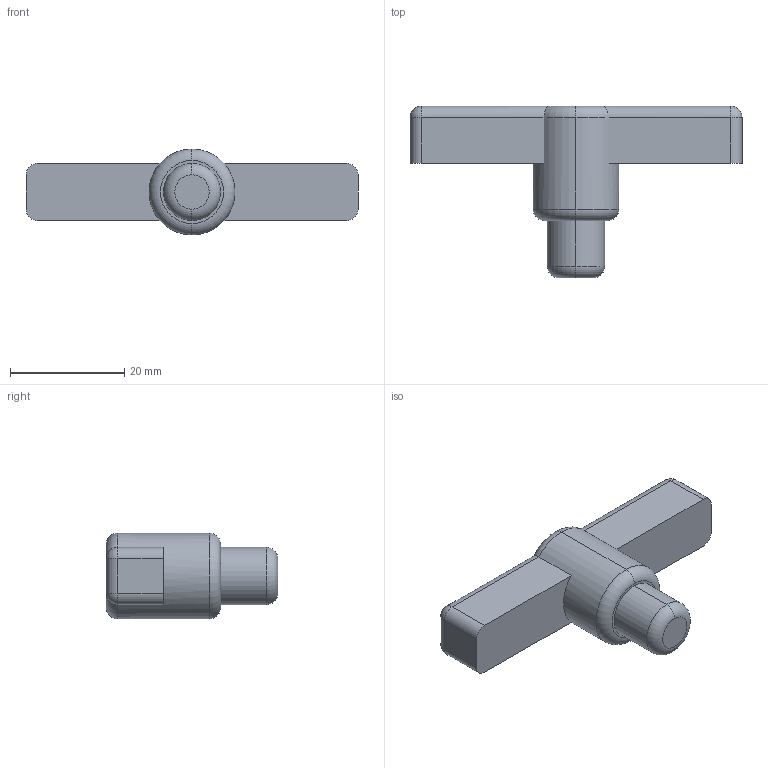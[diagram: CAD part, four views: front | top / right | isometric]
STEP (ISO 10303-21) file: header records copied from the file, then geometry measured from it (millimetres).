
FILE_DESCRIPTION (( 'STEP AP214' ), '1' );
FILE_NAME ('key.STEP', '2013-12-22T02:49:33', ( '' ), ( '' ), 'SwSTEP 2.0', 'SolidWorks 2013', '' );
FILE_SCHEMA (( 'AUTOMOTIVE_DESIGN' ));
Length unit declared in the file: millimetre
Products named in the file (1): key
Bounding box: 58 x 30 x 15 mm (x, y, z)
Volume: 8528.9 mm3; surface area: 3181.4 mm2
Topology: 1 solids, 1 shells, 36 faces, 82 edges, 45 vertices
Faces by surface type: cylinder 14, plane 11, torus 7, sphere 4
Entity records: 1052 total; most frequent: CARTESIAN_POINT 212, DIRECTION 188, ORIENTED_EDGE 156, EDGE_CURVE 78, AXIS2_PLACEMENT_3D 77, VERTEX_POINT 45, CIRCLE 40, EDGE_LOOP 37
